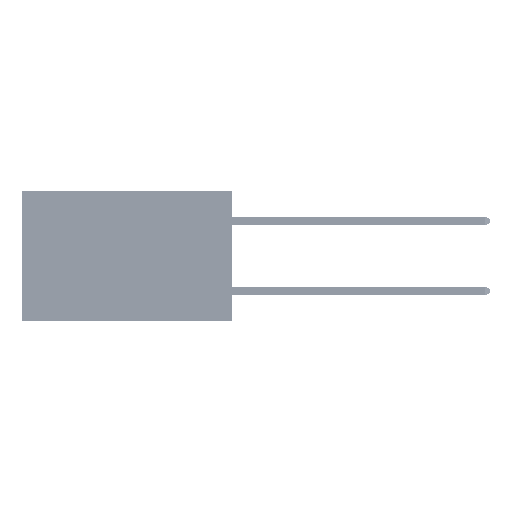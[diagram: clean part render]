
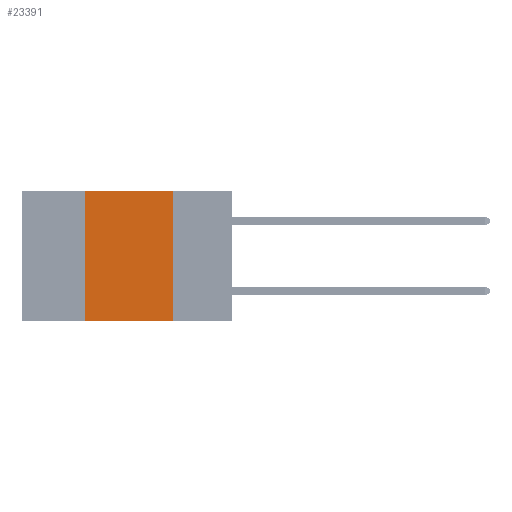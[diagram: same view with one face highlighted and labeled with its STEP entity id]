
A CAD part, left-side view. The second image highlights one B-rep face of the part: STEP entity #23391.
In plain terms, the highlighted planar face has unit normal (-1, 0, 0).
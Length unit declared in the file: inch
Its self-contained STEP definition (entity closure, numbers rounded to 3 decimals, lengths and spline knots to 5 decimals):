
#274 = CARTESIAN_POINT ( 'NONE',  ( 0., 0.6, 0. ) ) ;
#716 = EDGE_CURVE ( 'NONE', #16104, #25579, #42275, .T. ) ;
#2298 = ORIENTED_EDGE ( 'NONE', *, *, #716, .T. ) ;
#2535 = VECTOR ( 'NONE', #4911, 39.37008 ) ;
#3276 = VECTOR ( 'NONE', #46112, 39.37008 ) ;
#4911 = DIRECTION ( 'NONE',  ( 0., 0., 1. ) ) ;
#9547 = DIRECTION ( 'NONE',  ( 0., 0., -1. ) ) ;
#9765 = CARTESIAN_POINT ( 'NONE',  ( 0., 0.42, -0.37 ) ) ;
#10934 = CARTESIAN_POINT ( 'NONE',  ( 0., 0.6, 0. ) ) ;
#16073 = ORIENTED_EDGE ( 'NONE', *, *, #47178, .F. ) ;
#16104 = VERTEX_POINT ( 'NONE', #9765 ) ;
#17858 = AXIS2_PLACEMENT_3D ( 'NONE', #274, #43502, #20225 ) ;
#20225 = DIRECTION ( 'NONE',  ( 0., 0., -1. ) ) ;
#21876 = CARTESIAN_POINT ( 'NONE',  ( 0., 0.6, -0.37 ) ) ;
#23068 = ORIENTED_EDGE ( 'NONE', *, *, #23870, .F. ) ;
#23391 = ADVANCED_FACE ( 'NONE', ( #44261 ), #24622, .F. ) ;
#23870 = EDGE_CURVE ( 'NONE', #28638, #25579, #44980, .T. ) ;
#24587 = LINE ( 'NONE', #40336, #2535 ) ;
#24622 = PLANE ( 'NONE',  #17858 ) ;
#25579 = VERTEX_POINT ( 'NONE', #28394 ) ;
#26133 = VECTOR ( 'NONE', #9547, 39.37008 ) ;
#26231 = VECTOR ( 'NONE', #45407, 39.37008 ) ;
#26299 = CARTESIAN_POINT ( 'NONE',  ( 0., 0.42, 0. ) ) ;
#28007 = ORIENTED_EDGE ( 'NONE', *, *, #39874, .F. ) ;
#28394 = CARTESIAN_POINT ( 'NONE',  ( 0., 0.17, -0.37 ) ) ;
#28638 = VERTEX_POINT ( 'NONE', #47821 ) ;
#30646 = EDGE_LOOP ( 'NONE', ( #23068, #16073, #28007, #2298 ) ) ;
#33353 = CARTESIAN_POINT ( 'NONE',  ( 0., 0.17, 0. ) ) ;
#35463 = VERTEX_POINT ( 'NONE', #26299 ) ;
#39874 = EDGE_CURVE ( 'NONE', #16104, #35463, #24587, .T. ) ;
#40336 = CARTESIAN_POINT ( 'NONE',  ( 0., 0.42, 0. ) ) ;
#42275 = LINE ( 'NONE', #21876, #26231 ) ;
#43502 = DIRECTION ( 'NONE',  ( 1., 0., 0. ) ) ;
#44261 = FACE_OUTER_BOUND ( 'NONE', #30646, .T. ) ;
#44980 = LINE ( 'NONE', #33353, #26133 ) ;
#45407 = DIRECTION ( 'NONE',  ( 0., -1., 0. ) ) ;
#46112 = DIRECTION ( 'NONE',  ( 0., -1., 0. ) ) ;
#46368 = LINE ( 'NONE', #10934, #3276 ) ;
#47178 = EDGE_CURVE ( 'NONE', #35463, #28638, #46368, .T. ) ;
#47821 = CARTESIAN_POINT ( 'NONE',  ( 0., 0.17, 0. ) ) ;
